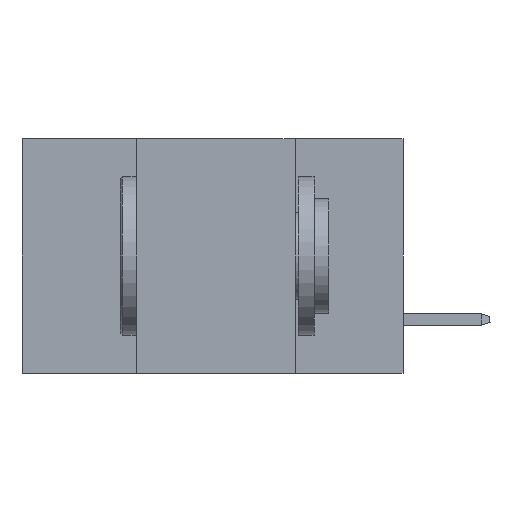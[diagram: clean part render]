
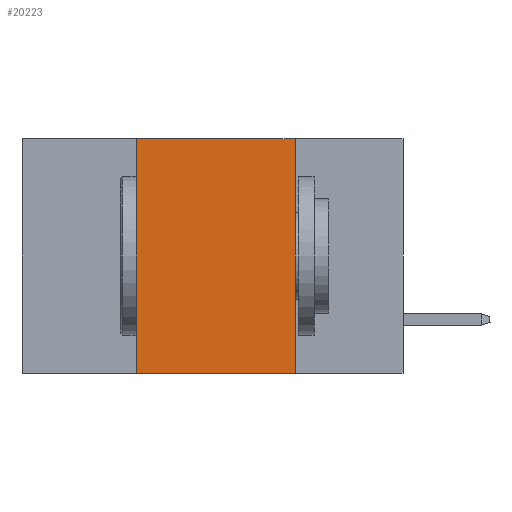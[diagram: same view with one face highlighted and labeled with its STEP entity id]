
A CAD part, left-side view. The second image highlights one B-rep face of the part: STEP entity #20223.
In plain terms, the highlighted planar face has unit normal (-1, 0, 0).
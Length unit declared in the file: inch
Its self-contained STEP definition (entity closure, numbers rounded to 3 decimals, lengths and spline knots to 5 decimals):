
#873 = CARTESIAN_POINT ( 'NONE',  ( 0., 0.6, 0. ) ) ;
#1555 = VERTEX_POINT ( 'NONE', #10810 ) ;
#2435 = CARTESIAN_POINT ( 'NONE',  ( 0., 0.17, 0. ) ) ;
#2544 = EDGE_CURVE ( 'NONE', #9571, #1555, #24870, .T. ) ;
#3481 = CARTESIAN_POINT ( 'NONE',  ( 0., 0.42, -0.37 ) ) ;
#4041 = CARTESIAN_POINT ( 'NONE',  ( 0., 0.17, 0. ) ) ;
#4233 = VECTOR ( 'NONE', #26560, 39.37008 ) ;
#5131 = ORIENTED_EDGE ( 'NONE', *, *, #10560, .F. ) ;
#5137 = VECTOR ( 'NONE', #23120, 39.37008 ) ;
#5319 = VERTEX_POINT ( 'NONE', #4041 ) ;
#5694 = VECTOR ( 'NONE', #9215, 39.37008 ) ;
#8933 = FACE_OUTER_BOUND ( 'NONE', #13326, .T. ) ;
#9215 = DIRECTION ( 'NONE',  ( 0., 0., 1. ) ) ;
#9273 = ORIENTED_EDGE ( 'NONE', *, *, #2544, .T. ) ;
#9571 = VERTEX_POINT ( 'NONE', #3481 ) ;
#10560 = EDGE_CURVE ( 'NONE', #5319, #1555, #18242, .T. ) ;
#10810 = CARTESIAN_POINT ( 'NONE',  ( 0., 0.17, -0.37 ) ) ;
#11314 = LINE ( 'NONE', #13918, #5694 ) ;
#13326 = EDGE_LOOP ( 'NONE', ( #5131, #22787, #23341, #9273 ) ) ;
#13662 = CARTESIAN_POINT ( 'NONE',  ( 0., 0.6, 0. ) ) ;
#13918 = CARTESIAN_POINT ( 'NONE',  ( 0., 0.42, 0. ) ) ;
#13961 = DIRECTION ( 'NONE',  ( 1., 0., 0. ) ) ;
#15652 = DIRECTION ( 'NONE',  ( 0., 0., -1. ) ) ;
#16174 = EDGE_CURVE ( 'NONE', #9571, #25724, #11314, .T. ) ;
#16994 = VECTOR ( 'NONE', #26845, 39.37008 ) ;
#17590 = CARTESIAN_POINT ( 'NONE',  ( 0., 0.6, -0.37 ) ) ;
#17951 = AXIS2_PLACEMENT_3D ( 'NONE', #13662, #13961, #15652 ) ;
#18242 = LINE ( 'NONE', #2435, #5137 ) ;
#20223 = ADVANCED_FACE ( 'NONE', ( #8933 ), #20632, .F. ) ;
#20632 = PLANE ( 'NONE',  #17951 ) ;
#22141 = LINE ( 'NONE', #873, #4233 ) ;
#22787 = ORIENTED_EDGE ( 'NONE', *, *, #28373, .F. ) ;
#23120 = DIRECTION ( 'NONE',  ( 0., 0., -1. ) ) ;
#23341 = ORIENTED_EDGE ( 'NONE', *, *, #16174, .F. ) ;
#24101 = CARTESIAN_POINT ( 'NONE',  ( 0., 0.42, 0. ) ) ;
#24870 = LINE ( 'NONE', #17590, #16994 ) ;
#25724 = VERTEX_POINT ( 'NONE', #24101 ) ;
#26560 = DIRECTION ( 'NONE',  ( 0., -1., 0. ) ) ;
#26845 = DIRECTION ( 'NONE',  ( 0., -1., 0. ) ) ;
#28373 = EDGE_CURVE ( 'NONE', #25724, #5319, #22141, .T. ) ;
